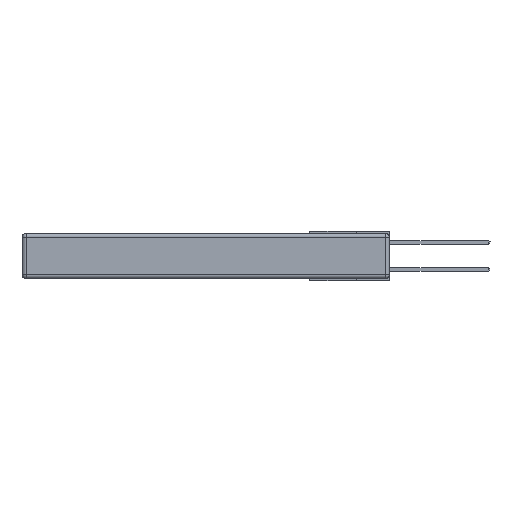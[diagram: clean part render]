
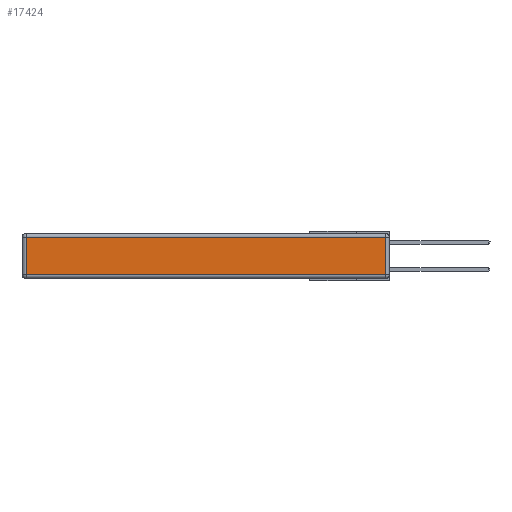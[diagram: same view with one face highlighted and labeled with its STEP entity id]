
A CAD part, left-side view. The second image highlights one B-rep face of the part: STEP entity #17424.
In plain terms, the highlighted planar face has unit normal (-1, 0, 0).
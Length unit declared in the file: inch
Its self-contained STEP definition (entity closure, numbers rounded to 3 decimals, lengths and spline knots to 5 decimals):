
#210 = CARTESIAN_POINT ( 'NONE',  ( 0., 2.72, -0.03 ) ) ;
#621 = CARTESIAN_POINT ( 'NONE',  ( 0., 2.72, -0.313 ) ) ;
#853 = ORIENTED_EDGE ( 'NONE', *, *, #5815, .T. ) ;
#2191 = AXIS2_PLACEMENT_3D ( 'NONE', #27182, #16233, #5112 ) ;
#4118 = CARTESIAN_POINT ( 'NONE',  ( 0., 2.75, -0.03 ) ) ;
#5112 = DIRECTION ( 'NONE',  ( 0., 0., 1. ) ) ;
#5229 = LINE ( 'NONE', #27495, #9705 ) ;
#5815 = EDGE_CURVE ( 'NONE', #15418, #6649, #27836, .T. ) ;
#5918 = LINE ( 'NONE', #17148, #6229 ) ;
#6207 = FACE_OUTER_BOUND ( 'NONE', #6292, .T. ) ;
#6229 = VECTOR ( 'NONE', #10460, 39.37008 ) ;
#6292 = EDGE_LOOP ( 'NONE', ( #20983, #21905, #853, #25991 ) ) ;
#6649 = VERTEX_POINT ( 'NONE', #210 ) ;
#7444 = PLANE ( 'NONE',  #2191 ) ;
#9263 = DIRECTION ( 'NONE',  ( 0., -1., 0. ) ) ;
#9705 = VECTOR ( 'NONE', #14270, 39.37008 ) ;
#9993 = LINE ( 'NONE', #15864, #17875 ) ;
#10460 = DIRECTION ( 'NONE',  ( 0., 0., -1. ) ) ;
#11296 = VERTEX_POINT ( 'NONE', #621 ) ;
#12017 = VERTEX_POINT ( 'NONE', #13089 ) ;
#13089 = CARTESIAN_POINT ( 'NONE',  ( 0., 0.03, -0.313 ) ) ;
#13178 = VECTOR ( 'NONE', #21708, 39.37008 ) ;
#14270 = DIRECTION ( 'NONE',  ( 0., 0., 1. ) ) ;
#15418 = VERTEX_POINT ( 'NONE', #15612 ) ;
#15612 = CARTESIAN_POINT ( 'NONE',  ( 0., 0.03, -0.03 ) ) ;
#15864 = CARTESIAN_POINT ( 'NONE',  ( 0., 0., -0.313 ) ) ;
#16233 = DIRECTION ( 'NONE',  ( -1., 0., 0. ) ) ;
#16802 = EDGE_CURVE ( 'NONE', #12017, #15418, #5229, .T. ) ;
#17148 = CARTESIAN_POINT ( 'NONE',  ( 0., 2.72, -0.343 ) ) ;
#17246 = EDGE_CURVE ( 'NONE', #11296, #12017, #9993, .T. ) ;
#17424 = ADVANCED_FACE ( 'NONE', ( #6207 ), #7444, .T. ) ;
#17875 = VECTOR ( 'NONE', #9263, 39.37008 ) ;
#20983 = ORIENTED_EDGE ( 'NONE', *, *, #17246, .T. ) ;
#21708 = DIRECTION ( 'NONE',  ( 0., 1., 0. ) ) ;
#21905 = ORIENTED_EDGE ( 'NONE', *, *, #16802, .T. ) ;
#25387 = EDGE_CURVE ( 'NONE', #6649, #11296, #5918, .T. ) ;
#25991 = ORIENTED_EDGE ( 'NONE', *, *, #25387, .T. ) ;
#27182 = CARTESIAN_POINT ( 'NONE',  ( 0., 0., -0.343 ) ) ;
#27495 = CARTESIAN_POINT ( 'NONE',  ( 0., 0.03, -0.343 ) ) ;
#27836 = LINE ( 'NONE', #4118, #13178 ) ;
